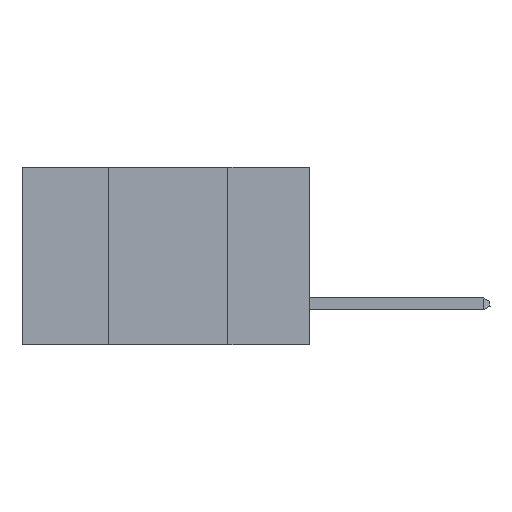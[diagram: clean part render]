
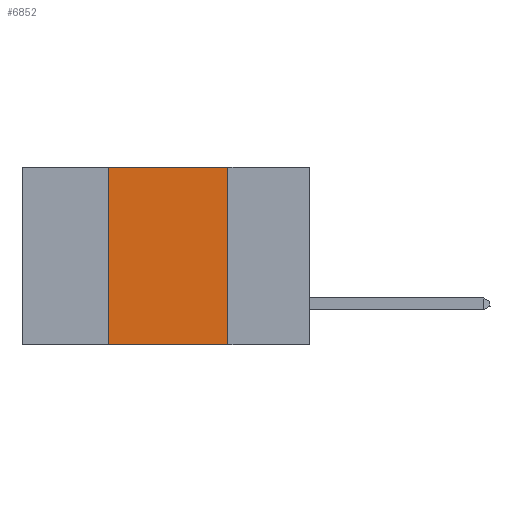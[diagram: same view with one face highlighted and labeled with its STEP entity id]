
A CAD part, left-side view. The second image highlights one B-rep face of the part: STEP entity #6852.
In plain terms, the highlighted planar face has unit normal (-1, 0, 0).
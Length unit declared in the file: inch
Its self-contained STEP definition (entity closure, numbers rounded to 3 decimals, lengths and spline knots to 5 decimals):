
#12 = DIRECTION ( 'NONE',  ( 0., -1., 0. ) ) ;
#222 = CARTESIAN_POINT ( 'NONE',  ( 0., 0.6, -0.37 ) ) ;
#268 = ORIENTED_EDGE ( 'NONE', *, *, #8345, .F. ) ;
#459 = VECTOR ( 'NONE', #6278, 39.37008 ) ;
#953 = DIRECTION ( 'NONE',  ( 1., 0., 0. ) ) ;
#1103 = AXIS2_PLACEMENT_3D ( 'NONE', #6008, #953, #3186 ) ;
#1877 = VECTOR ( 'NONE', #4166, 39.37008 ) ;
#1930 = EDGE_CURVE ( 'NONE', #8195, #4618, #3043, .T. ) ;
#2006 = VERTEX_POINT ( 'NONE', #4192 ) ;
#2569 = EDGE_CURVE ( 'NONE', #8195, #11061, #4129, .T. ) ;
#2722 = VECTOR ( 'NONE', #10964, 39.37008 ) ;
#3043 = LINE ( 'NONE', #222, #8442 ) ;
#3186 = DIRECTION ( 'NONE',  ( 0., 0., -1. ) ) ;
#3328 = CARTESIAN_POINT ( 'NONE',  ( 0., 0.42, 0. ) ) ;
#3534 = LINE ( 'NONE', #9884, #2722 ) ;
#3660 = ORIENTED_EDGE ( 'NONE', *, *, #1930, .T. ) ;
#3725 = ORIENTED_EDGE ( 'NONE', *, *, #3877, .F. ) ;
#3877 = EDGE_CURVE ( 'NONE', #11061, #2006, #8882, .T. ) ;
#4129 = LINE ( 'NONE', #9371, #459 ) ;
#4166 = DIRECTION ( 'NONE',  ( 0., -1., 0. ) ) ;
#4192 = CARTESIAN_POINT ( 'NONE',  ( 0., 0.17, 0. ) ) ;
#4618 = VERTEX_POINT ( 'NONE', #10841 ) ;
#6008 = CARTESIAN_POINT ( 'NONE',  ( 0., 0.6, 0. ) ) ;
#6145 = CARTESIAN_POINT ( 'NONE',  ( 0., 0.6, 0. ) ) ;
#6173 = PLANE ( 'NONE',  #1103 ) ;
#6278 = DIRECTION ( 'NONE',  ( 0., 0., 1. ) ) ;
#6710 = FACE_OUTER_BOUND ( 'NONE', #8784, .T. ) ;
#6852 = ADVANCED_FACE ( 'NONE', ( #6710 ), #6173, .F. ) ;
#7190 = ORIENTED_EDGE ( 'NONE', *, *, #2569, .F. ) ;
#8195 = VERTEX_POINT ( 'NONE', #12637 ) ;
#8345 = EDGE_CURVE ( 'NONE', #2006, #4618, #3534, .T. ) ;
#8442 = VECTOR ( 'NONE', #12, 39.37008 ) ;
#8784 = EDGE_LOOP ( 'NONE', ( #268, #3725, #7190, #3660 ) ) ;
#8882 = LINE ( 'NONE', #6145, #1877 ) ;
#9371 = CARTESIAN_POINT ( 'NONE',  ( 0., 0.42, 0. ) ) ;
#9884 = CARTESIAN_POINT ( 'NONE',  ( 0., 0.17, 0. ) ) ;
#10841 = CARTESIAN_POINT ( 'NONE',  ( 0., 0.17, -0.37 ) ) ;
#10964 = DIRECTION ( 'NONE',  ( 0., 0., -1. ) ) ;
#11061 = VERTEX_POINT ( 'NONE', #3328 ) ;
#12637 = CARTESIAN_POINT ( 'NONE',  ( 0., 0.42, -0.37 ) ) ;
